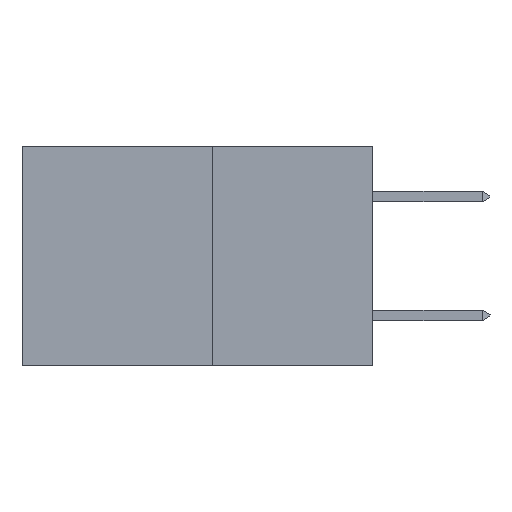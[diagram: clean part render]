
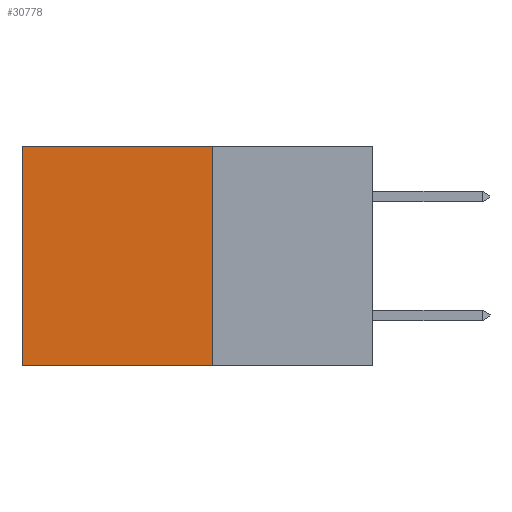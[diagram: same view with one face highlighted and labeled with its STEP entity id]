
A CAD part, left-side view. The second image highlights one B-rep face of the part: STEP entity #30778.
In plain terms, the highlighted planar face has unit normal (-1, 0, 0).
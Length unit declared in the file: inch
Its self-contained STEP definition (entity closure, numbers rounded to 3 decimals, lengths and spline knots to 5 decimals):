
#98 = FACE_OUTER_BOUND ( 'NONE', #29923, .T. ) ;
#1188 = ORIENTED_EDGE ( 'NONE', *, *, #9941, .F. ) ;
#1902 = CARTESIAN_POINT ( 'NONE',  ( 0.277, 0.27, 0. ) ) ;
#2286 = ORIENTED_EDGE ( 'NONE', *, *, #16135, .T. ) ;
#4061 = EDGE_CURVE ( 'NONE', #9704, #16548, #33382, .T. ) ;
#4481 = CARTESIAN_POINT ( 'NONE',  ( 0.277, 0.27, -0.37 ) ) ;
#4554 = VECTOR ( 'NONE', #26586, 39.37008 ) ;
#5020 = DIRECTION ( 'NONE',  ( 0., 1., 0. ) ) ;
#6280 = CARTESIAN_POINT ( 'NONE',  ( 0.277, 0.27, 0. ) ) ;
#9287 = VECTOR ( 'NONE', #18185, 39.37008 ) ;
#9320 = PLANE ( 'NONE',  #35016 ) ;
#9704 = VERTEX_POINT ( 'NONE', #11832 ) ;
#9941 = EDGE_CURVE ( 'NONE', #33804, #9704, #33987, .T. ) ;
#11832 = CARTESIAN_POINT ( 'NONE',  ( 0.277, 0.27, -0.37 ) ) ;
#12114 = DIRECTION ( 'NONE',  ( 0., 0., -1. ) ) ;
#15342 = VECTOR ( 'NONE', #22814, 39.37008 ) ;
#15443 = CARTESIAN_POINT ( 'NONE',  ( 0.277, 0.59, -0.37 ) ) ;
#16135 = EDGE_CURVE ( 'NONE', #33804, #30999, #21767, .T. ) ;
#16548 = VERTEX_POINT ( 'NONE', #32838 ) ;
#18185 = DIRECTION ( 'NONE',  ( 0., 0., -1. ) ) ;
#20717 = EDGE_CURVE ( 'NONE', #30999, #16548, #31325, .T. ) ;
#21767 = LINE ( 'NONE', #6280, #15342 ) ;
#22458 = ORIENTED_EDGE ( 'NONE', *, *, #20717, .T. ) ;
#22814 = DIRECTION ( 'NONE',  ( 0., 1., 0. ) ) ;
#23201 = ORIENTED_EDGE ( 'NONE', *, *, #4061, .F. ) ;
#23765 = CARTESIAN_POINT ( 'NONE',  ( 0.277, 0.27, -0.37 ) ) ;
#24531 = CARTESIAN_POINT ( 'NONE',  ( 0.277, 0.59, 0. ) ) ;
#25892 = CARTESIAN_POINT ( 'NONE',  ( 0.277, 0.27, -0.37 ) ) ;
#26056 = VECTOR ( 'NONE', #5020, 39.37008 ) ;
#26586 = DIRECTION ( 'NONE',  ( 0., 0., -1. ) ) ;
#28684 = DIRECTION ( 'NONE',  ( 1., 0., 0. ) ) ;
#29923 = EDGE_LOOP ( 'NONE', ( #22458, #23201, #1188, #2286 ) ) ;
#30778 = ADVANCED_FACE ( 'NONE', ( #98 ), #9320, .F. ) ;
#30999 = VERTEX_POINT ( 'NONE', #24531 ) ;
#31325 = LINE ( 'NONE', #15443, #9287 ) ;
#32838 = CARTESIAN_POINT ( 'NONE',  ( 0.277, 0.59, -0.37 ) ) ;
#33382 = LINE ( 'NONE', #4481, #26056 ) ;
#33804 = VERTEX_POINT ( 'NONE', #1902 ) ;
#33987 = LINE ( 'NONE', #23765, #4554 ) ;
#35016 = AXIS2_PLACEMENT_3D ( 'NONE', #25892, #28684, #12114 ) ;
